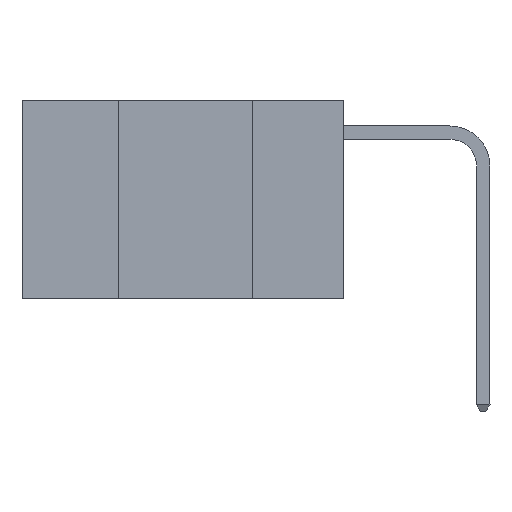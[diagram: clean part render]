
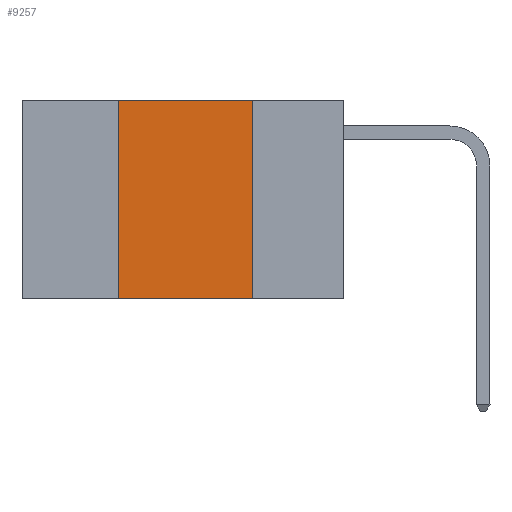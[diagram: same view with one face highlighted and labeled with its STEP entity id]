
A CAD part, left-side view. The second image highlights one B-rep face of the part: STEP entity #9257.
In plain terms, the highlighted planar face has unit normal (-1, 0, 0).
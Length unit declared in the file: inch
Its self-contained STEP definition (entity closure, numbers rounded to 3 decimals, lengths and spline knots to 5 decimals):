
#1076 = EDGE_LOOP ( 'NONE', ( #12237, #16915, #22533, #20907 ) ) ;
#3129 = EDGE_CURVE ( 'NONE', #3297, #6752, #19944, .T. ) ;
#3297 = VERTEX_POINT ( 'NONE', #5220 ) ;
#4515 = CARTESIAN_POINT ( 'NONE',  ( 0., 0.17, -0.37 ) ) ;
#5071 = CARTESIAN_POINT ( 'NONE',  ( 0., 0.17, 0. ) ) ;
#5220 = CARTESIAN_POINT ( 'NONE',  ( 0., 0.42, 0. ) ) ;
#6752 = VERTEX_POINT ( 'NONE', #5071 ) ;
#6893 = CARTESIAN_POINT ( 'NONE',  ( 0., 0.6, 0. ) ) ;
#8900 = AXIS2_PLACEMENT_3D ( 'NONE', #6893, #16959, #10836 ) ;
#9257 = ADVANCED_FACE ( 'NONE', ( #10963 ), #11335, .F. ) ;
#9819 = CARTESIAN_POINT ( 'NONE',  ( 0., 0.17, 0. ) ) ;
#10822 = CARTESIAN_POINT ( 'NONE',  ( 0., 0.6, -0.37 ) ) ;
#10836 = DIRECTION ( 'NONE',  ( 0., 0., -1. ) ) ;
#10876 = VECTOR ( 'NONE', #14311, 39.37008 ) ;
#10963 = FACE_OUTER_BOUND ( 'NONE', #1076, .T. ) ;
#11128 = CARTESIAN_POINT ( 'NONE',  ( 0., 0.42, -0.37 ) ) ;
#11335 = PLANE ( 'NONE',  #8900 ) ;
#12237 = ORIENTED_EDGE ( 'NONE', *, *, #20687, .F. ) ;
#12369 = CARTESIAN_POINT ( 'NONE',  ( 0., 0.6, 0. ) ) ;
#13521 = DIRECTION ( 'NONE',  ( 0., 0., -1. ) ) ;
#14079 = EDGE_CURVE ( 'NONE', #23000, #19100, #22880, .T. ) ;
#14311 = DIRECTION ( 'NONE',  ( 0., 0., 1. ) ) ;
#14776 = VECTOR ( 'NONE', #13521, 39.37008 ) ;
#15228 = VECTOR ( 'NONE', #22138, 39.37008 ) ;
#16915 = ORIENTED_EDGE ( 'NONE', *, *, #3129, .F. ) ;
#16959 = DIRECTION ( 'NONE',  ( 1., 0., 0. ) ) ;
#17094 = VECTOR ( 'NONE', #20688, 39.37008 ) ;
#18653 = CARTESIAN_POINT ( 'NONE',  ( 0., 0.42, 0. ) ) ;
#19100 = VERTEX_POINT ( 'NONE', #4515 ) ;
#19944 = LINE ( 'NONE', #12369, #15228 ) ;
#20687 = EDGE_CURVE ( 'NONE', #6752, #19100, #25044, .T. ) ;
#20688 = DIRECTION ( 'NONE',  ( 0., -1., 0. ) ) ;
#20907 = ORIENTED_EDGE ( 'NONE', *, *, #14079, .T. ) ;
#22138 = DIRECTION ( 'NONE',  ( 0., -1., 0. ) ) ;
#22533 = ORIENTED_EDGE ( 'NONE', *, *, #25012, .F. ) ;
#22880 = LINE ( 'NONE', #10822, #17094 ) ;
#23000 = VERTEX_POINT ( 'NONE', #11128 ) ;
#24056 = LINE ( 'NONE', #18653, #10876 ) ;
#25012 = EDGE_CURVE ( 'NONE', #23000, #3297, #24056, .T. ) ;
#25044 = LINE ( 'NONE', #9819, #14776 ) ;
